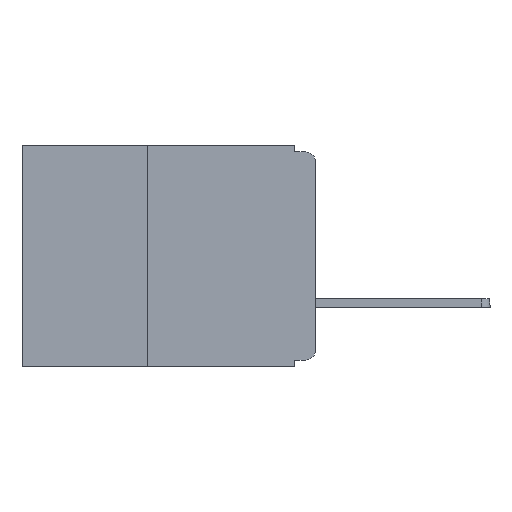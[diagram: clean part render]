
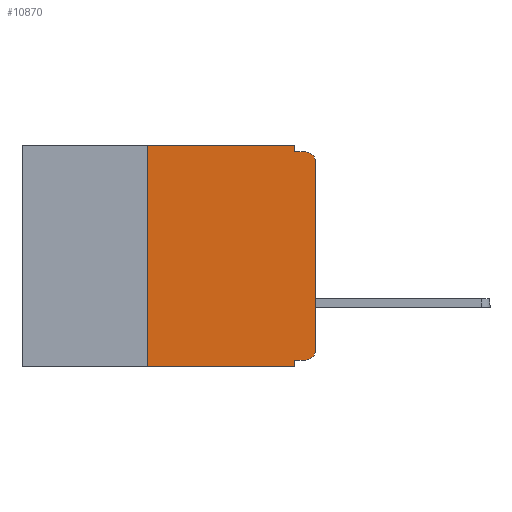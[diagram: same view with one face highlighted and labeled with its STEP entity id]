
A CAD part, left-side view. The second image highlights one B-rep face of the part: STEP entity #10870.
In plain terms, the highlighted planar face has unit normal (-1, 0, 0).
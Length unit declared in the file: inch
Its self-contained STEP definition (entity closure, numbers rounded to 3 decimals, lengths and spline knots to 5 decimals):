
#389 = ORIENTED_EDGE ( 'NONE', *, *, #455, .F. ) ;
#407 = LINE ( 'NONE', #7026, #11623 ) ;
#411 = CARTESIAN_POINT ( 'NONE',  ( 0., 0.031, -0.33 ) ) ;
#455 = EDGE_CURVE ( 'NONE', #4952, #5744, #407, .T. ) ;
#463 = VERTEX_POINT ( 'NONE', #4218 ) ;
#487 = EDGE_CURVE ( 'NONE', #11732, #3789, #11189, .T. ) ;
#522 = EDGE_CURVE ( 'NONE', #11732, #2116, #11087, .T. ) ;
#542 = EDGE_CURVE ( 'NONE', #7336, #2116, #10981, .T. ) ;
#604 = ORIENTED_EDGE ( 'NONE', *, *, #10536, .F. ) ;
#711 = VECTOR ( 'NONE', #4989, 39.37008 ) ;
#790 = LINE ( 'NONE', #11208, #711 ) ;
#1101 = CARTESIAN_POINT ( 'NONE',  ( 0., 0., -0.305 ) ) ;
#1264 = ORIENTED_EDGE ( 'NONE', *, *, #487, .F. ) ;
#1311 = ORIENTED_EDGE ( 'NONE', *, *, #522, .T. ) ;
#1354 = ORIENTED_EDGE ( 'NONE', *, *, #4135, .F. ) ;
#1392 = CIRCLE ( 'NONE', #8900, 0.015 ) ;
#1656 = ORIENTED_EDGE ( 'NONE', *, *, #542, .F. ) ;
#1768 = CARTESIAN_POINT ( 'NONE',  ( 0., 0.015, -0.32 ) ) ;
#1913 = ORIENTED_EDGE ( 'NONE', *, *, #10659, .T. ) ;
#2072 = ORIENTED_EDGE ( 'NONE', *, *, #3017, .T. ) ;
#2116 = VERTEX_POINT ( 'NONE', #411 ) ;
#2668 = CARTESIAN_POINT ( 'NONE',  ( 0., 0.437, -0.33 ) ) ;
#2677 = ORIENTED_EDGE ( 'NONE', *, *, #4219, .F. ) ;
#3017 = EDGE_CURVE ( 'NONE', #7653, #3714, #790, .T. ) ;
#3213 = ORIENTED_EDGE ( 'NONE', *, *, #4259, .T. ) ;
#3216 = CARTESIAN_POINT ( 'NONE',  ( 0., 0.031, -0.33 ) ) ;
#3409 = DIRECTION ( 'NONE',  ( 0., -1., 0. ) ) ;
#3450 = CARTESIAN_POINT ( 'NONE',  ( 0., 0., -0.01 ) ) ;
#3461 = DIRECTION ( 'NONE',  ( 0., 0., -1. ) ) ;
#3714 = VERTEX_POINT ( 'NONE', #10640 ) ;
#3789 = VERTEX_POINT ( 'NONE', #4980 ) ;
#3983 = DIRECTION ( 'NONE',  ( -1., 0., 0. ) ) ;
#4135 = EDGE_CURVE ( 'NONE', #5744, #463, #9670, .T. ) ;
#4159 = DIRECTION ( 'NONE',  ( 0., 0., -1. ) ) ;
#4172 = DIRECTION ( 'NONE',  ( 0., 0., -1. ) ) ;
#4218 = CARTESIAN_POINT ( 'NONE',  ( 0., 0.015, -0.01 ) ) ;
#4219 = EDGE_CURVE ( 'NONE', #5727, #7336, #9283, .T. ) ;
#4259 = EDGE_CURVE ( 'NONE', #5727, #7653, #9095, .T. ) ;
#4536 = DIRECTION ( 'NONE',  ( -1., 0., 0. ) ) ;
#4600 = CARTESIAN_POINT ( 'NONE',  ( 0., 0.015, -0.305 ) ) ;
#4952 = VERTEX_POINT ( 'NONE', #11423 ) ;
#4980 = CARTESIAN_POINT ( 'NONE',  ( 0., 0.25, 0. ) ) ;
#4989 = DIRECTION ( 'NONE',  ( 0., 0., 1. ) ) ;
#5222 = CARTESIAN_POINT ( 'NONE',  ( 0., 0.031, -0.32 ) ) ;
#5309 = PLANE ( 'NONE',  #8635 ) ;
#5399 = VECTOR ( 'NONE', #5711, 39.37008 ) ;
#5711 = DIRECTION ( 'NONE',  ( 0., -1., 0. ) ) ;
#5727 = VERTEX_POINT ( 'NONE', #1768 ) ;
#5744 = VERTEX_POINT ( 'NONE', #11172 ) ;
#7026 = CARTESIAN_POINT ( 'NONE',  ( 0., 0.031, 0. ) ) ;
#7291 = DIRECTION ( 'NONE',  ( 0., 0., -1. ) ) ;
#7336 = VERTEX_POINT ( 'NONE', #5222 ) ;
#7546 = CARTESIAN_POINT ( 'NONE',  ( 0., 0.25, -0.33 ) ) ;
#7653 = VERTEX_POINT ( 'NONE', #1101 ) ;
#7699 = DIRECTION ( 'NONE',  ( 1., 0., 0. ) ) ;
#7701 = CARTESIAN_POINT ( 'NONE',  ( 0., 0.25, -0.33 ) ) ;
#8019 = LINE ( 'NONE', #10916, #5399 ) ;
#8155 = AXIS2_PLACEMENT_3D ( 'NONE', #4600, #4536, #4159 ) ;
#8254 = CARTESIAN_POINT ( 'NONE',  ( 0., 0., -0.32 ) ) ;
#8635 = AXIS2_PLACEMENT_3D ( 'NONE', #11298, #7699, #7291 ) ;
#8853 = FACE_OUTER_BOUND ( 'NONE', #9265, .T. ) ;
#8900 = AXIS2_PLACEMENT_3D ( 'NONE', #9656, #3983, #10388 ) ;
#9095 = CIRCLE ( 'NONE', #8155, 0.015 ) ;
#9262 = VECTOR ( 'NONE', #10075, 39.37008 ) ;
#9265 = EDGE_LOOP ( 'NONE', ( #2072, #1913, #1354, #389, #604, #1264, #1311, #1656, #2677, #3213 ) ) ;
#9283 = LINE ( 'NONE', #8254, #9262 ) ;
#9650 = VECTOR ( 'NONE', #3409, 39.37008 ) ;
#9656 = CARTESIAN_POINT ( 'NONE',  ( 0., 0.015, -0.025 ) ) ;
#9670 = LINE ( 'NONE', #3450, #9650 ) ;
#10075 = DIRECTION ( 'NONE',  ( 0., 1., 0. ) ) ;
#10292 = DIRECTION ( 'NONE',  ( 0., 0., 1. ) ) ;
#10388 = DIRECTION ( 'NONE',  ( 0., 0., -1. ) ) ;
#10536 = EDGE_CURVE ( 'NONE', #3789, #4952, #8019, .T. ) ;
#10640 = CARTESIAN_POINT ( 'NONE',  ( 0., 0., -0.025 ) ) ;
#10659 = EDGE_CURVE ( 'NONE', #3714, #463, #1392, .T. ) ;
#10730 = DIRECTION ( 'NONE',  ( 0., -1., 0. ) ) ;
#10870 = ADVANCED_FACE ( 'NONE', ( #8853 ), #5309, .F. ) ;
#10916 = CARTESIAN_POINT ( 'NONE',  ( 0., 0.437, 0. ) ) ;
#10981 = LINE ( 'NONE', #3216, #11177 ) ;
#11078 = VECTOR ( 'NONE', #10730, 39.37008 ) ;
#11087 = LINE ( 'NONE', #2668, #11078 ) ;
#11164 = VECTOR ( 'NONE', #10292, 39.37008 ) ;
#11172 = CARTESIAN_POINT ( 'NONE',  ( 0., 0.031, -0.01 ) ) ;
#11177 = VECTOR ( 'NONE', #3461, 39.37008 ) ;
#11189 = LINE ( 'NONE', #7546, #11164 ) ;
#11208 = CARTESIAN_POINT ( 'NONE',  ( 0., 0., 0. ) ) ;
#11298 = CARTESIAN_POINT ( 'NONE',  ( 0., 0.437, 0. ) ) ;
#11423 = CARTESIAN_POINT ( 'NONE',  ( 0., 0.031, 0. ) ) ;
#11623 = VECTOR ( 'NONE', #4172, 39.37008 ) ;
#11732 = VERTEX_POINT ( 'NONE', #7701 ) ;
